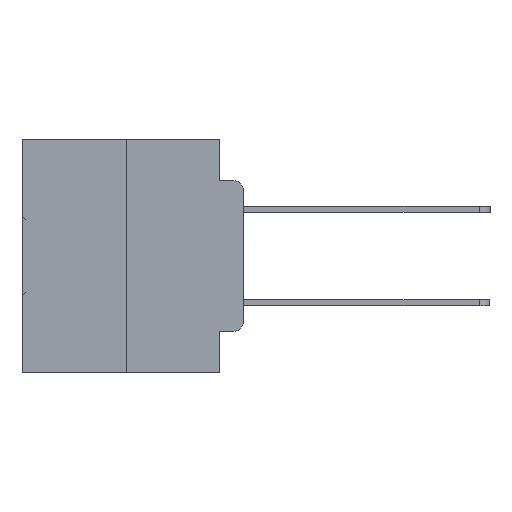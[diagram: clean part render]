
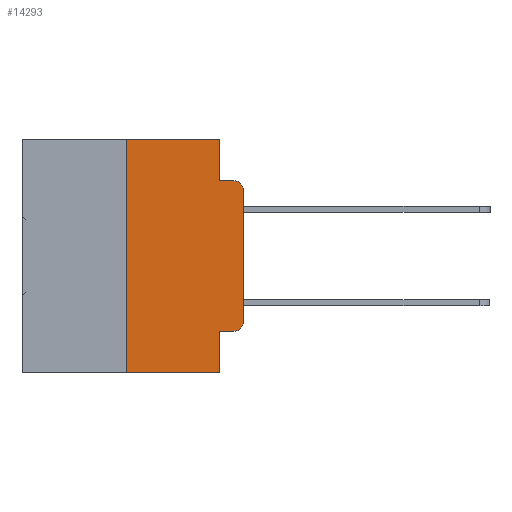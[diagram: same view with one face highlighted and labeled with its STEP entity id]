
A CAD part, left-side view. The second image highlights one B-rep face of the part: STEP entity #14293.
In plain terms, the highlighted planar face has unit normal (-1, 0, 0).
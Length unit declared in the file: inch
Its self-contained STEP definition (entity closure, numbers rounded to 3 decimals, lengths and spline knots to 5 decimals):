
#626 = DIRECTION ( 'NONE',  ( 0., 0., -1. ) ) ;
#1334 = ORIENTED_EDGE ( 'NONE', *, *, #22245, .T. ) ;
#1383 = CARTESIAN_POINT ( 'NONE',  ( 0., 0.473, 0. ) ) ;
#2016 = VERTEX_POINT ( 'NONE', #11593 ) ;
#2059 = DIRECTION ( 'NONE',  ( 0., 0., -1. ) ) ;
#3014 = CARTESIAN_POINT ( 'NONE',  ( 0., 0.02, -0.3915 ) ) ;
#3073 = VERTEX_POINT ( 'NONE', #12044 ) ;
#3296 = CARTESIAN_POINT ( 'NONE',  ( 0., 0., 0. ) ) ;
#5714 = VECTOR ( 'NONE', #10844, 39.37008 ) ;
#5750 = DIRECTION ( 'NONE',  ( 0., 0., -1. ) ) ;
#6562 = VERTEX_POINT ( 'NONE', #18451 ) ;
#6712 = VECTOR ( 'NONE', #15773, 39.37008 ) ;
#7264 = CARTESIAN_POINT ( 'NONE',  ( 0., 0.25, -0.5 ) ) ;
#7402 = CARTESIAN_POINT ( 'NONE',  ( 0., 0.02, -0.4115 ) ) ;
#7515 = VECTOR ( 'NONE', #16484, 39.37008 ) ;
#7516 = VECTOR ( 'NONE', #626, 39.37008 ) ;
#7814 = VERTEX_POINT ( 'NONE', #7264 ) ;
#8724 = DIRECTION ( 'NONE',  ( 0., 0., 1. ) ) ;
#8753 = CARTESIAN_POINT ( 'NONE',  ( 0., 0.25, 0. ) ) ;
#8814 = AXIS2_PLACEMENT_3D ( 'NONE', #34014, #18162, #2059 ) ;
#9352 = LINE ( 'NONE', #21750, #23665 ) ;
#10272 = ORIENTED_EDGE ( 'NONE', *, *, #12469, .T. ) ;
#10318 = VECTOR ( 'NONE', #25579, 39.37008 ) ;
#10395 = CARTESIAN_POINT ( 'NONE',  ( 0., 0.02, -0.1085 ) ) ;
#10844 = DIRECTION ( 'NONE',  ( 0., -1., 0. ) ) ;
#11369 = CIRCLE ( 'NONE', #18225, 0.02 ) ;
#11593 = CARTESIAN_POINT ( 'NONE',  ( 0., 0., -0.1085 ) ) ;
#12044 = CARTESIAN_POINT ( 'NONE',  ( 0., 0.051, -0.5 ) ) ;
#12469 = EDGE_CURVE ( 'NONE', #2016, #13062, #11369, .T. ) ;
#12718 = CARTESIAN_POINT ( 'NONE',  ( 0., 0.02, -0.0885 ) ) ;
#12823 = VECTOR ( 'NONE', #26051, 39.37008 ) ;
#13054 = CARTESIAN_POINT ( 'NONE',  ( 0., 0.051, 0. ) ) ;
#13062 = VERTEX_POINT ( 'NONE', #12718 ) ;
#13109 = DIRECTION ( 'NONE',  ( 0., 0., -1. ) ) ;
#13569 = CARTESIAN_POINT ( 'NONE',  ( 0., 0.051, -0.4115 ) ) ;
#14293 = ADVANCED_FACE ( 'NONE', ( #17562 ), #15441, .F. ) ;
#14457 = ORIENTED_EDGE ( 'NONE', *, *, #23127, .F. ) ;
#14645 = LINE ( 'NONE', #21777, #7515 ) ;
#14648 = LINE ( 'NONE', #32658, #7516 ) ;
#15441 = PLANE ( 'NONE',  #8814 ) ;
#15773 = DIRECTION ( 'NONE',  ( 0., 0., -1. ) ) ;
#15862 = EDGE_LOOP ( 'NONE', ( #32054, #10272, #30317, #31558, #16138, #28250, #19509, #14457, #19070, #1334 ) ) ;
#16138 = ORIENTED_EDGE ( 'NONE', *, *, #24573, .F. ) ;
#16484 = DIRECTION ( 'NONE',  ( 0., -1., 0. ) ) ;
#16746 = VERTEX_POINT ( 'NONE', #18130 ) ;
#16830 = EDGE_CURVE ( 'NONE', #23319, #16746, #21852, .T. ) ;
#17562 = FACE_OUTER_BOUND ( 'NONE', #15862, .T. ) ;
#17964 = CARTESIAN_POINT ( 'NONE',  ( 0., 0.25, 0. ) ) ;
#18130 = CARTESIAN_POINT ( 'NONE',  ( 0., 0.051, -0.0885 ) ) ;
#18162 = DIRECTION ( 'NONE',  ( 1., 0., 0. ) ) ;
#18225 = AXIS2_PLACEMENT_3D ( 'NONE', #10395, #29109, #13109 ) ;
#18451 = CARTESIAN_POINT ( 'NONE',  ( 0., 0., -0.3915 ) ) ;
#19070 = ORIENTED_EDGE ( 'NONE', *, *, #24928, .T. ) ;
#19509 = ORIENTED_EDGE ( 'NONE', *, *, #21742, .T. ) ;
#19988 = LINE ( 'NONE', #17964, #12823 ) ;
#20133 = VERTEX_POINT ( 'NONE', #25712 ) ;
#20182 = CIRCLE ( 'NONE', #27837, 0.02 ) ;
#20844 = LINE ( 'NONE', #13569, #5714 ) ;
#21574 = LINE ( 'NONE', #3296, #26980 ) ;
#21742 = EDGE_CURVE ( 'NONE', #7814, #3073, #9352, .T. ) ;
#21750 = CARTESIAN_POINT ( 'NONE',  ( 0., 0.473, -0.5 ) ) ;
#21777 = CARTESIAN_POINT ( 'NONE',  ( 0., 0.051, -0.0885 ) ) ;
#21834 = DIRECTION ( 'NONE',  ( -1., 0., 0. ) ) ;
#21852 = LINE ( 'NONE', #13054, #6712 ) ;
#22245 = EDGE_CURVE ( 'NONE', #32246, #6562, #20182, .T. ) ;
#23127 = EDGE_CURVE ( 'NONE', #20133, #3073, #14648, .T. ) ;
#23153 = VERTEX_POINT ( 'NONE', #8753 ) ;
#23319 = VERTEX_POINT ( 'NONE', #30779 ) ;
#23665 = VECTOR ( 'NONE', #26981, 39.37008 ) ;
#24573 = EDGE_CURVE ( 'NONE', #23153, #23319, #24658, .T. ) ;
#24658 = LINE ( 'NONE', #1383, #10318 ) ;
#24928 = EDGE_CURVE ( 'NONE', #20133, #32246, #20844, .T. ) ;
#25579 = DIRECTION ( 'NONE',  ( 0., -1., 0. ) ) ;
#25712 = CARTESIAN_POINT ( 'NONE',  ( 0., 0.051, -0.4115 ) ) ;
#26051 = DIRECTION ( 'NONE',  ( 0., 0., 1. ) ) ;
#26980 = VECTOR ( 'NONE', #8724, 39.37008 ) ;
#26981 = DIRECTION ( 'NONE',  ( 0., -1., 0. ) ) ;
#27837 = AXIS2_PLACEMENT_3D ( 'NONE', #3014, #21834, #5750 ) ;
#28250 = ORIENTED_EDGE ( 'NONE', *, *, #32214, .F. ) ;
#28603 = EDGE_CURVE ( 'NONE', #6562, #2016, #21574, .T. ) ;
#29109 = DIRECTION ( 'NONE',  ( -1., 0., 0. ) ) ;
#30317 = ORIENTED_EDGE ( 'NONE', *, *, #30381, .F. ) ;
#30381 = EDGE_CURVE ( 'NONE', #16746, #13062, #14645, .T. ) ;
#30779 = CARTESIAN_POINT ( 'NONE',  ( 0., 0.051, 0. ) ) ;
#31558 = ORIENTED_EDGE ( 'NONE', *, *, #16830, .F. ) ;
#32054 = ORIENTED_EDGE ( 'NONE', *, *, #28603, .T. ) ;
#32214 = EDGE_CURVE ( 'NONE', #7814, #23153, #19988, .T. ) ;
#32246 = VERTEX_POINT ( 'NONE', #7402 ) ;
#32658 = CARTESIAN_POINT ( 'NONE',  ( 0., 0.051, 0. ) ) ;
#34014 = CARTESIAN_POINT ( 'NONE',  ( 0., 0.473, 0. ) ) ;
